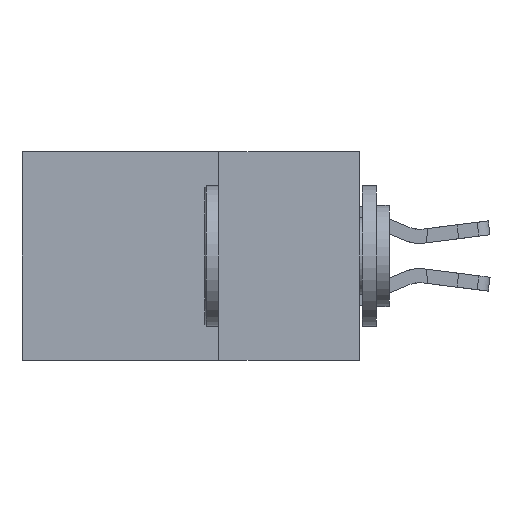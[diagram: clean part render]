
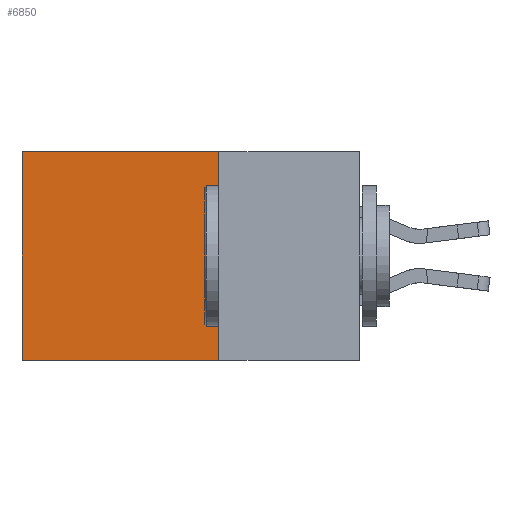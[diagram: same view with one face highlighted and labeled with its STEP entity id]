
A CAD part, left-side view. The second image highlights one B-rep face of the part: STEP entity #6850.
In plain terms, the highlighted planar face has unit normal (-1, 0, 0).
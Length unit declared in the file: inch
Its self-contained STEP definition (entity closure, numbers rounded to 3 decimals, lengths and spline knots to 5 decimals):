
#206 = CARTESIAN_POINT ( 'NONE',  ( 0.2875, 0.25, 0. ) ) ;
#598 = DIRECTION ( 'NONE',  ( 1., 0., 0. ) ) ;
#1084 = LINE ( 'NONE', #3958, #15755 ) ;
#1173 = CARTESIAN_POINT ( 'NONE',  ( 0.2875, 0.6, -0.37 ) ) ;
#2181 = VECTOR ( 'NONE', #8685, 39.37008 ) ;
#2695 = EDGE_LOOP ( 'NONE', ( #4755, #13743, #12049, #3162 ) ) ;
#2737 = VERTEX_POINT ( 'NONE', #13089 ) ;
#3050 = LINE ( 'NONE', #17432, #3522 ) ;
#3162 = ORIENTED_EDGE ( 'NONE', *, *, #14346, .T. ) ;
#3522 = VECTOR ( 'NONE', #9150, 39.37008 ) ;
#3958 = CARTESIAN_POINT ( 'NONE',  ( 0.2875, 0.25, -0.37 ) ) ;
#4453 = VERTEX_POINT ( 'NONE', #15066 ) ;
#4755 = ORIENTED_EDGE ( 'NONE', *, *, #9891, .T. ) ;
#5068 = CARTESIAN_POINT ( 'NONE',  ( 0.2875, 0.25, 0. ) ) ;
#5182 = FACE_OUTER_BOUND ( 'NONE', #2695, .T. ) ;
#5395 = VERTEX_POINT ( 'NONE', #206 ) ;
#5572 = EDGE_CURVE ( 'NONE', #5395, #2737, #11764, .T. ) ;
#5802 = VERTEX_POINT ( 'NONE', #1173 ) ;
#6850 = ADVANCED_FACE ( 'NONE', ( #5182 ), #7878, .F. ) ;
#7878 = PLANE ( 'NONE',  #15425 ) ;
#8047 = VECTOR ( 'NONE', #9333, 39.37008 ) ;
#8213 = DIRECTION ( 'NONE',  ( 0., 1., 0. ) ) ;
#8685 = DIRECTION ( 'NONE',  ( 0., 1., 0. ) ) ;
#9150 = DIRECTION ( 'NONE',  ( 0., 0., -1. ) ) ;
#9333 = DIRECTION ( 'NONE',  ( 0., 0., -1. ) ) ;
#9891 = EDGE_CURVE ( 'NONE', #4453, #5802, #3050, .T. ) ;
#10688 = DIRECTION ( 'NONE',  ( 0., 0., -1. ) ) ;
#11287 = EDGE_CURVE ( 'NONE', #2737, #5802, #1084, .T. ) ;
#11764 = LINE ( 'NONE', #5068, #8047 ) ;
#12049 = ORIENTED_EDGE ( 'NONE', *, *, #5572, .F. ) ;
#13089 = CARTESIAN_POINT ( 'NONE',  ( 0.2875, 0.25, -0.37 ) ) ;
#13743 = ORIENTED_EDGE ( 'NONE', *, *, #11287, .F. ) ;
#14346 = EDGE_CURVE ( 'NONE', #5395, #4453, #17574, .T. ) ;
#15066 = CARTESIAN_POINT ( 'NONE',  ( 0.2875, 0.6, 0. ) ) ;
#15425 = AXIS2_PLACEMENT_3D ( 'NONE', #17570, #598, #10688 ) ;
#15755 = VECTOR ( 'NONE', #8213, 39.37008 ) ;
#17432 = CARTESIAN_POINT ( 'NONE',  ( 0.2875, 0.6, 0. ) ) ;
#17434 = CARTESIAN_POINT ( 'NONE',  ( 0.2875, 0.25, 0. ) ) ;
#17570 = CARTESIAN_POINT ( 'NONE',  ( 0.2875, 0.25, 0. ) ) ;
#17574 = LINE ( 'NONE', #17434, #2181 ) ;
